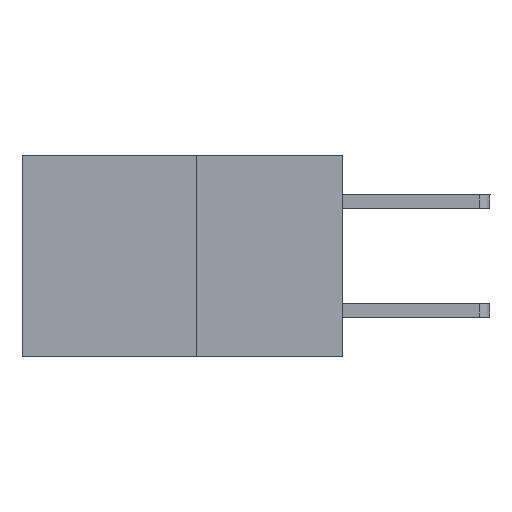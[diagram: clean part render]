
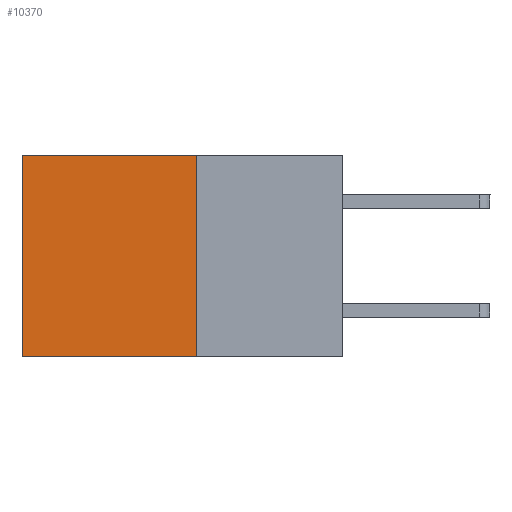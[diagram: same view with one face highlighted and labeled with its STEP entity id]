
A CAD part, left-side view. The second image highlights one B-rep face of the part: STEP entity #10370.
In plain terms, the highlighted planar face has unit normal (-1, 0, 0).
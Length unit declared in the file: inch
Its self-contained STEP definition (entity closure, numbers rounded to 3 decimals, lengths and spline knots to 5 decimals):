
#19 = ORIENTED_EDGE ( 'NONE', *, *, #2360, .T. ) ;
#262 = VERTEX_POINT ( 'NONE', #7635 ) ;
#323 = LINE ( 'NONE', #2100, #11286 ) ;
#557 = VECTOR ( 'NONE', #6797, 39.37008 ) ;
#1897 = VERTEX_POINT ( 'NONE', #3782 ) ;
#2100 = CARTESIAN_POINT ( 'NONE',  ( 0.277, 0.27, -0.37 ) ) ;
#2360 = EDGE_CURVE ( 'NONE', #1897, #7754, #10892, .T. ) ;
#2409 = CARTESIAN_POINT ( 'NONE',  ( 0.277, 0.27, 0. ) ) ;
#2465 = LINE ( 'NONE', #6014, #9662 ) ;
#2509 = DIRECTION ( 'NONE',  ( 0., 0., -1. ) ) ;
#3411 = VERTEX_POINT ( 'NONE', #2409 ) ;
#3481 = EDGE_CURVE ( 'NONE', #3411, #1897, #2465, .T. ) ;
#3782 = CARTESIAN_POINT ( 'NONE',  ( 0.277, 0.59, 0. ) ) ;
#4145 = DIRECTION ( 'NONE',  ( 0., 1., 0. ) ) ;
#5245 = ORIENTED_EDGE ( 'NONE', *, *, #3481, .T. ) ;
#5506 = EDGE_LOOP ( 'NONE', ( #19, #8772, #8942, #5245 ) ) ;
#6014 = CARTESIAN_POINT ( 'NONE',  ( 0.277, 0.27, 0. ) ) ;
#6337 = CARTESIAN_POINT ( 'NONE',  ( 0.277, 0.59, -0.37 ) ) ;
#6785 = VECTOR ( 'NONE', #7317, 39.37008 ) ;
#6797 = DIRECTION ( 'NONE',  ( 0., 0., -1. ) ) ;
#6843 = AXIS2_PLACEMENT_3D ( 'NONE', #11309, #10440, #2509 ) ;
#6934 = FACE_OUTER_BOUND ( 'NONE', #5506, .T. ) ;
#7317 = DIRECTION ( 'NONE',  ( 0., 0., -1. ) ) ;
#7469 = CARTESIAN_POINT ( 'NONE',  ( 0.277, 0.59, -0.37 ) ) ;
#7608 = CARTESIAN_POINT ( 'NONE',  ( 0.277, 0.27, -0.37 ) ) ;
#7635 = CARTESIAN_POINT ( 'NONE',  ( 0.277, 0.27, -0.37 ) ) ;
#7722 = LINE ( 'NONE', #7608, #557 ) ;
#7754 = VERTEX_POINT ( 'NONE', #7469 ) ;
#8673 = PLANE ( 'NONE',  #6843 ) ;
#8772 = ORIENTED_EDGE ( 'NONE', *, *, #10042, .F. ) ;
#8942 = ORIENTED_EDGE ( 'NONE', *, *, #9247, .F. ) ;
#9181 = DIRECTION ( 'NONE',  ( 0., 1., 0. ) ) ;
#9247 = EDGE_CURVE ( 'NONE', #3411, #262, #7722, .T. ) ;
#9662 = VECTOR ( 'NONE', #4145, 39.37008 ) ;
#10042 = EDGE_CURVE ( 'NONE', #262, #7754, #323, .T. ) ;
#10370 = ADVANCED_FACE ( 'NONE', ( #6934 ), #8673, .F. ) ;
#10440 = DIRECTION ( 'NONE',  ( 1., 0., 0. ) ) ;
#10892 = LINE ( 'NONE', #6337, #6785 ) ;
#11286 = VECTOR ( 'NONE', #9181, 39.37008 ) ;
#11309 = CARTESIAN_POINT ( 'NONE',  ( 0.277, 0.27, -0.37 ) ) ;
